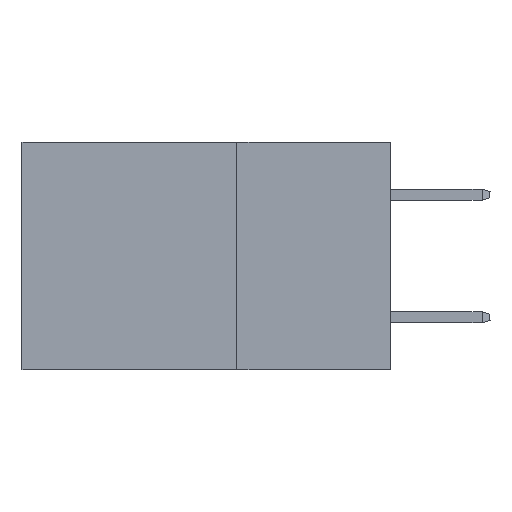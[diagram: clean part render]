
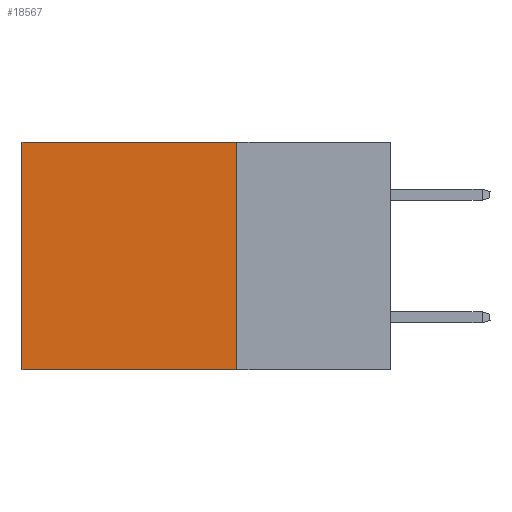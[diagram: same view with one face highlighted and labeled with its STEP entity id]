
A CAD part, left-side view. The second image highlights one B-rep face of the part: STEP entity #18567.
In plain terms, the highlighted planar face has unit normal (-1, 0, 0).
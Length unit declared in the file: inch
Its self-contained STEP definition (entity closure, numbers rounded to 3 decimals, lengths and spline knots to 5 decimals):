
#559 = CARTESIAN_POINT ( 'NONE',  ( 0.2875, 0.6, 0. ) ) ;
#1561 = DIRECTION ( 'NONE',  ( 0., 0., -1. ) ) ;
#2028 = CARTESIAN_POINT ( 'NONE',  ( 0.2875, 0.25, 0. ) ) ;
#2497 = DIRECTION ( 'NONE',  ( 0., 0., -1. ) ) ;
#3181 = CARTESIAN_POINT ( 'NONE',  ( 0.2875, 0.25, 0. ) ) ;
#3894 = LINE ( 'NONE', #6671, #18014 ) ;
#4395 = LINE ( 'NONE', #5817, #5009 ) ;
#5009 = VECTOR ( 'NONE', #22211, 39.37008 ) ;
#5399 = EDGE_CURVE ( 'NONE', #18576, #6124, #4395, .T. ) ;
#5817 = CARTESIAN_POINT ( 'NONE',  ( 0.2875, 0.25, -0.37 ) ) ;
#6124 = VERTEX_POINT ( 'NONE', #20975 ) ;
#6671 = CARTESIAN_POINT ( 'NONE',  ( 0.2875, 0.25, 0. ) ) ;
#6920 = FACE_OUTER_BOUND ( 'NONE', #9274, .T. ) ;
#7129 = LINE ( 'NONE', #559, #21074 ) ;
#7137 = CARTESIAN_POINT ( 'NONE',  ( 0.2875, 0.25, 0. ) ) ;
#7207 = PLANE ( 'NONE',  #20881 ) ;
#8399 = LINE ( 'NONE', #2028, #16957 ) ;
#9274 = EDGE_LOOP ( 'NONE', ( #16217, #15249, #23094, #21774 ) ) ;
#11400 = VERTEX_POINT ( 'NONE', #3181 ) ;
#12270 = DIRECTION ( 'NONE',  ( 0., 0., -1. ) ) ;
#12772 = DIRECTION ( 'NONE',  ( 1., 0., 0. ) ) ;
#12941 = EDGE_CURVE ( 'NONE', #11400, #14579, #8399, .T. ) ;
#14363 = CARTESIAN_POINT ( 'NONE',  ( 0.2875, 0.6, 0. ) ) ;
#14579 = VERTEX_POINT ( 'NONE', #14363 ) ;
#15249 = ORIENTED_EDGE ( 'NONE', *, *, #5399, .F. ) ;
#16217 = ORIENTED_EDGE ( 'NONE', *, *, #20077, .T. ) ;
#16785 = DIRECTION ( 'NONE',  ( 0., 1., 0. ) ) ;
#16957 = VECTOR ( 'NONE', #16785, 39.37008 ) ;
#18014 = VECTOR ( 'NONE', #12270, 39.37008 ) ;
#18567 = ADVANCED_FACE ( 'NONE', ( #6920 ), #7207, .F. ) ;
#18576 = VERTEX_POINT ( 'NONE', #20021 ) ;
#19551 = EDGE_CURVE ( 'NONE', #11400, #18576, #3894, .T. ) ;
#20021 = CARTESIAN_POINT ( 'NONE',  ( 0.2875, 0.25, -0.37 ) ) ;
#20077 = EDGE_CURVE ( 'NONE', #14579, #6124, #7129, .T. ) ;
#20881 = AXIS2_PLACEMENT_3D ( 'NONE', #7137, #12772, #1561 ) ;
#20975 = CARTESIAN_POINT ( 'NONE',  ( 0.2875, 0.6, -0.37 ) ) ;
#21074 = VECTOR ( 'NONE', #2497, 39.37008 ) ;
#21774 = ORIENTED_EDGE ( 'NONE', *, *, #12941, .T. ) ;
#22211 = DIRECTION ( 'NONE',  ( 0., 1., 0. ) ) ;
#23094 = ORIENTED_EDGE ( 'NONE', *, *, #19551, .F. ) ;
